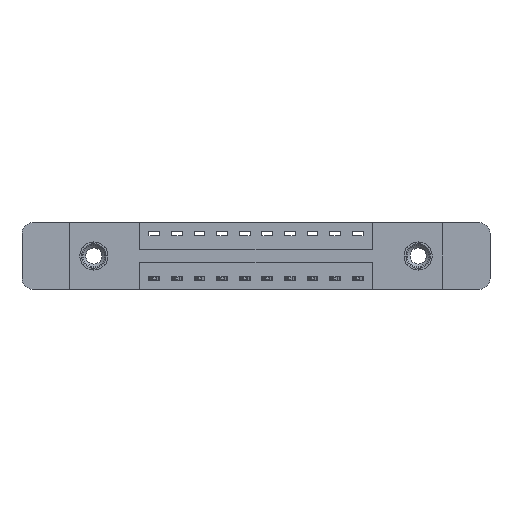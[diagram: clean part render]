
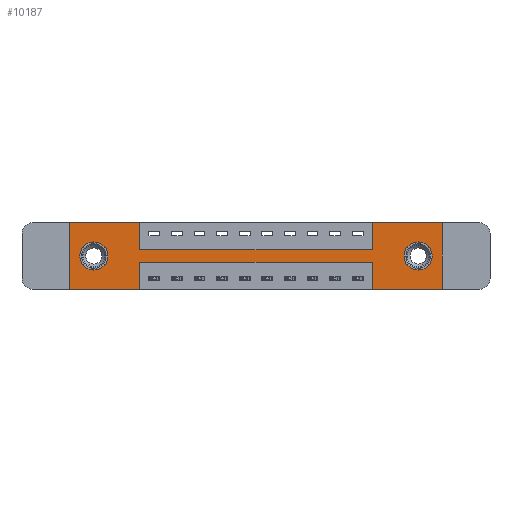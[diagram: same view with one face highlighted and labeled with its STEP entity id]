
A CAD part, front view. The second image highlights one B-rep face of the part: STEP entity #10187.
In plain terms, the highlighted planar face has unit normal (0, -1, 0).
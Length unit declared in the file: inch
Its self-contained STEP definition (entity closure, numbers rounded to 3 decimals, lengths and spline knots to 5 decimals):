
#211 = AXIS2_PLACEMENT_3D ( 'NONE', #10054, #5320, #6622 ) ;
#513 = LINE ( 'NONE', #13295, #1591 ) ;
#556 = EDGE_CURVE ( 'NONE', #12697, #6796, #2857, .T. ) ;
#634 = CARTESIAN_POINT ( 'NONE',  ( 0., 0., -0.37 ) ) ;
#806 = LINE ( 'NONE', #7191, #8385 ) ;
#861 = EDGE_CURVE ( 'NONE', #10966, #9930, #8945, .T. ) ;
#988 = CARTESIAN_POINT ( 'NONE',  ( 1.6725, 0., 0. ) ) ;
#1128 = LINE ( 'NONE', #3500, #2269 ) ;
#1309 = DIRECTION ( 'NONE',  ( 1., 0., 0. ) ) ;
#1591 = VECTOR ( 'NONE', #7136, 39.37008 ) ;
#1656 = VECTOR ( 'NONE', #9470, 39.37008 ) ;
#1699 = ORIENTED_EDGE ( 'NONE', *, *, #4533, .F. ) ;
#1918 = EDGE_CURVE ( 'NONE', #6796, #9269, #11577, .T. ) ;
#2011 = CARTESIAN_POINT ( 'NONE',  ( 0.3875, 0., -0.22 ) ) ;
#2043 = CARTESIAN_POINT ( 'NONE',  ( 0., 0., -0.37 ) ) ;
#2075 = LINE ( 'NONE', #3978, #4921 ) ;
#2133 = EDGE_CURVE ( 'NONE', #9633, #5989, #1128, .T. ) ;
#2269 = VECTOR ( 'NONE', #4615, 39.37008 ) ;
#2428 = CARTESIAN_POINT ( 'NONE',  ( 0., 0., 0. ) ) ;
#2716 = CARTESIAN_POINT ( 'NONE',  ( 0.3875, 0., 0. ) ) ;
#2857 = LINE ( 'NONE', #3764, #9540 ) ;
#2955 = CARTESIAN_POINT ( 'NONE',  ( 0., 0., -0.37 ) ) ;
#3057 = VECTOR ( 'NONE', #10205, 39.37008 ) ;
#3111 = EDGE_CURVE ( 'NONE', #9930, #10966, #13094, .T. ) ;
#3134 = CARTESIAN_POINT ( 'NONE',  ( 2.06, 0., -0.37 ) ) ;
#3500 = CARTESIAN_POINT ( 'NONE',  ( 1.6725, 0., -0.37 ) ) ;
#3666 = ORIENTED_EDGE ( 'NONE', *, *, #5241, .T. ) ;
#3726 = CARTESIAN_POINT ( 'NONE',  ( 0.3875, 0., 0. ) ) ;
#3764 = CARTESIAN_POINT ( 'NONE',  ( 0., 0., 0. ) ) ;
#3850 = ORIENTED_EDGE ( 'NONE', *, *, #3111, .T. ) ;
#3865 = ORIENTED_EDGE ( 'NONE', *, *, #13986, .F. ) ;
#3918 = ORIENTED_EDGE ( 'NONE', *, *, #15525, .F. ) ;
#3978 = CARTESIAN_POINT ( 'NONE',  ( 1.6725, 0., 0. ) ) ;
#4082 = CARTESIAN_POINT ( 'NONE',  ( 0., 0., 0. ) ) ;
#4117 = ORIENTED_EDGE ( 'NONE', *, *, #861, .T. ) ;
#4146 = AXIS2_PLACEMENT_3D ( 'NONE', #5984, #9429, #9590 ) ;
#4371 = VERTEX_POINT ( 'NONE', #988 ) ;
#4533 = EDGE_CURVE ( 'NONE', #8673, #12697, #9724, .T. ) ;
#4564 = ORIENTED_EDGE ( 'NONE', *, *, #556, .F. ) ;
#4615 = DIRECTION ( 'NONE',  ( 0., 0., 1. ) ) ;
#4742 = CARTESIAN_POINT ( 'NONE',  ( 0.3875, 0., -0.37 ) ) ;
#4896 = AXIS2_PLACEMENT_3D ( 'NONE', #10311, #11487, #5495 ) ;
#4921 = VECTOR ( 'NONE', #13644, 39.37008 ) ;
#5202 = FACE_OUTER_BOUND ( 'NONE', #7495, .T. ) ;
#5241 = EDGE_CURVE ( 'NONE', #8832, #5950, #13333, .T. ) ;
#5307 = VECTOR ( 'NONE', #12779, 39.37008 ) ;
#5320 = DIRECTION ( 'NONE',  ( 0., 1., 0. ) ) ;
#5495 = DIRECTION ( 'NONE',  ( 0., 0., 1. ) ) ;
#5521 = CARTESIAN_POINT ( 'NONE',  ( 0.1325, 0., -0.185 ) ) ;
#5636 = VECTOR ( 'NONE', #15694, 39.37008 ) ;
#5754 = VECTOR ( 'NONE', #6633, 39.37008 ) ;
#5801 = CARTESIAN_POINT ( 'NONE',  ( 1.9275, 0., -0.263 ) ) ;
#5950 = VERTEX_POINT ( 'NONE', #14678 ) ;
#5984 = CARTESIAN_POINT ( 'NONE',  ( 1.9275, 0., -0.185 ) ) ;
#5989 = VERTEX_POINT ( 'NONE', #14070 ) ;
#6403 = EDGE_CURVE ( 'NONE', #5950, #8832, #7223, .T. ) ;
#6484 = VERTEX_POINT ( 'NONE', #2011 ) ;
#6553 = CARTESIAN_POINT ( 'NONE',  ( 0.3875, 0., -0.37 ) ) ;
#6569 = AXIS2_PLACEMENT_3D ( 'NONE', #5521, #14011, #9230 ) ;
#6622 = DIRECTION ( 'NONE',  ( 0., 0., -1. ) ) ;
#6633 = DIRECTION ( 'NONE',  ( 0., 0., 1. ) ) ;
#6796 = VERTEX_POINT ( 'NONE', #2716 ) ;
#6914 = VERTEX_POINT ( 'NONE', #3134 ) ;
#6924 = EDGE_CURVE ( 'NONE', #6914, #9633, #8347, .T. ) ;
#7136 = DIRECTION ( 'NONE',  ( -1., 0., 0. ) ) ;
#7191 = CARTESIAN_POINT ( 'NONE',  ( 0.3875, 0., -0.15 ) ) ;
#7223 = CIRCLE ( 'NONE', #6569, 0.078 ) ;
#7495 = EDGE_LOOP ( 'NONE', ( #12553, #10370, #13329, #7949, #11648, #10949, #3918, #9878, #15017, #4564, #1699, #3865 ) ) ;
#7949 = ORIENTED_EDGE ( 'NONE', *, *, #6924, .F. ) ;
#8250 = CARTESIAN_POINT ( 'NONE',  ( 2.06, 0., 0. ) ) ;
#8347 = LINE ( 'NONE', #634, #5307 ) ;
#8385 = VECTOR ( 'NONE', #10790, 39.37008 ) ;
#8387 = EDGE_LOOP ( 'NONE', ( #3850, #4117 ) ) ;
#8440 = DIRECTION ( 'NONE',  ( 0., 0., -1. ) ) ;
#8533 = VECTOR ( 'NONE', #8440, 39.37008 ) ;
#8673 = VERTEX_POINT ( 'NONE', #15375 ) ;
#8806 = FACE_BOUND ( 'NONE', #15428, .T. ) ;
#8832 = VERTEX_POINT ( 'NONE', #13249 ) ;
#8842 = LINE ( 'NONE', #15645, #5636 ) ;
#8930 = DIRECTION ( 'NONE',  ( 0., 0., -1. ) ) ;
#8945 = CIRCLE ( 'NONE', #4146, 0.078 ) ;
#9230 = DIRECTION ( 'NONE',  ( 0., 0., 1. ) ) ;
#9269 = VERTEX_POINT ( 'NONE', #13170 ) ;
#9357 = DIRECTION ( 'NONE',  ( 0., -1., 0. ) ) ;
#9429 = DIRECTION ( 'NONE',  ( 0., 1., 0. ) ) ;
#9470 = DIRECTION ( 'NONE',  ( 0., 0., -1. ) ) ;
#9540 = VECTOR ( 'NONE', #1309, 39.37008 ) ;
#9545 = LINE ( 'NONE', #2955, #3057 ) ;
#9587 = FACE_BOUND ( 'NONE', #8387, .T. ) ;
#9590 = DIRECTION ( 'NONE',  ( 0., 0., -1. ) ) ;
#9633 = VERTEX_POINT ( 'NONE', #12738 ) ;
#9724 = LINE ( 'NONE', #2428, #5754 ) ;
#9878 = ORIENTED_EDGE ( 'NONE', *, *, #10382, .F. ) ;
#9886 = VERTEX_POINT ( 'NONE', #11868 ) ;
#9900 = VERTEX_POINT ( 'NONE', #8250 ) ;
#9930 = VERTEX_POINT ( 'NONE', #10910 ) ;
#10054 = CARTESIAN_POINT ( 'NONE',  ( 1.9275, 0., -0.185 ) ) ;
#10187 = ADVANCED_FACE ( 'NONE', ( #9587, #8806, #5202 ), #14042, .T. ) ;
#10205 = DIRECTION ( 'NONE',  ( -1., 0., 0. ) ) ;
#10311 = CARTESIAN_POINT ( 'NONE',  ( 0.1325, 0., -0.185 ) ) ;
#10361 = EDGE_CURVE ( 'NONE', #6484, #10687, #11361, .T. ) ;
#10370 = ORIENTED_EDGE ( 'NONE', *, *, #10407, .F. ) ;
#10382 = EDGE_CURVE ( 'NONE', #9269, #9886, #806, .T. ) ;
#10407 = EDGE_CURVE ( 'NONE', #5989, #6484, #513, .T. ) ;
#10687 = VERTEX_POINT ( 'NONE', #6553 ) ;
#10790 = DIRECTION ( 'NONE',  ( 1., 0., 0. ) ) ;
#10910 = CARTESIAN_POINT ( 'NONE',  ( 1.9275, 0., -0.107 ) ) ;
#10949 = ORIENTED_EDGE ( 'NONE', *, *, #11731, .F. ) ;
#10966 = VERTEX_POINT ( 'NONE', #5801 ) ;
#11321 = CARTESIAN_POINT ( 'NONE',  ( 2.06, 0., 0. ) ) ;
#11361 = LINE ( 'NONE', #4742, #1656 ) ;
#11487 = DIRECTION ( 'NONE',  ( 0., 1., 0. ) ) ;
#11577 = LINE ( 'NONE', #3726, #8533 ) ;
#11648 = ORIENTED_EDGE ( 'NONE', *, *, #15083, .F. ) ;
#11731 = EDGE_CURVE ( 'NONE', #4371, #9900, #8842, .T. ) ;
#11747 = DIRECTION ( 'NONE',  ( 0., 0., -1. ) ) ;
#11758 = AXIS2_PLACEMENT_3D ( 'NONE', #2043, #9357, #11747 ) ;
#11868 = CARTESIAN_POINT ( 'NONE',  ( 1.6725, 0., -0.15 ) ) ;
#12168 = VECTOR ( 'NONE', #8930, 39.37008 ) ;
#12553 = ORIENTED_EDGE ( 'NONE', *, *, #10361, .F. ) ;
#12697 = VERTEX_POINT ( 'NONE', #4082 ) ;
#12738 = CARTESIAN_POINT ( 'NONE',  ( 1.6725, 0., -0.37 ) ) ;
#12779 = DIRECTION ( 'NONE',  ( -1., 0., 0. ) ) ;
#13094 = CIRCLE ( 'NONE', #211, 0.078 ) ;
#13170 = CARTESIAN_POINT ( 'NONE',  ( 0.3875, 0., -0.15 ) ) ;
#13249 = CARTESIAN_POINT ( 'NONE',  ( 0.1325, 0., -0.263 ) ) ;
#13295 = CARTESIAN_POINT ( 'NONE',  ( 0.3875, 0., -0.22 ) ) ;
#13312 = LINE ( 'NONE', #11321, #12168 ) ;
#13329 = ORIENTED_EDGE ( 'NONE', *, *, #2133, .F. ) ;
#13333 = CIRCLE ( 'NONE', #4896, 0.078 ) ;
#13644 = DIRECTION ( 'NONE',  ( 0., 0., 1. ) ) ;
#13986 = EDGE_CURVE ( 'NONE', #10687, #8673, #9545, .T. ) ;
#14011 = DIRECTION ( 'NONE',  ( 0., 1., 0. ) ) ;
#14042 = PLANE ( 'NONE',  #11758 ) ;
#14070 = CARTESIAN_POINT ( 'NONE',  ( 1.6725, 0., -0.22 ) ) ;
#14480 = ORIENTED_EDGE ( 'NONE', *, *, #6403, .T. ) ;
#14678 = CARTESIAN_POINT ( 'NONE',  ( 0.1325, 0., -0.107 ) ) ;
#15017 = ORIENTED_EDGE ( 'NONE', *, *, #1918, .F. ) ;
#15083 = EDGE_CURVE ( 'NONE', #9900, #6914, #13312, .T. ) ;
#15375 = CARTESIAN_POINT ( 'NONE',  ( 0., 0., -0.37 ) ) ;
#15428 = EDGE_LOOP ( 'NONE', ( #14480, #3666 ) ) ;
#15525 = EDGE_CURVE ( 'NONE', #9886, #4371, #2075, .T. ) ;
#15645 = CARTESIAN_POINT ( 'NONE',  ( 0., 0., 0. ) ) ;
#15694 = DIRECTION ( 'NONE',  ( 1., 0., 0. ) ) ;
